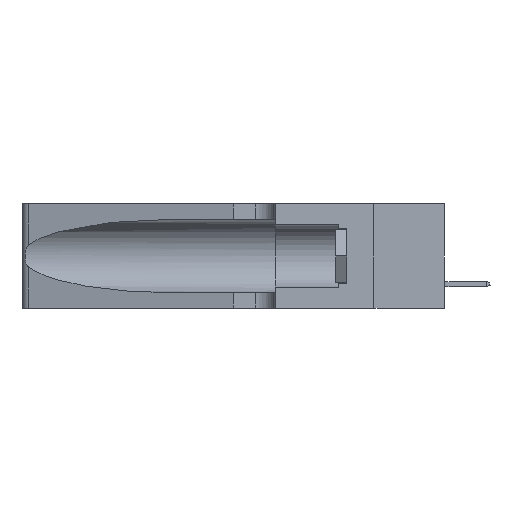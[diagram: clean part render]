
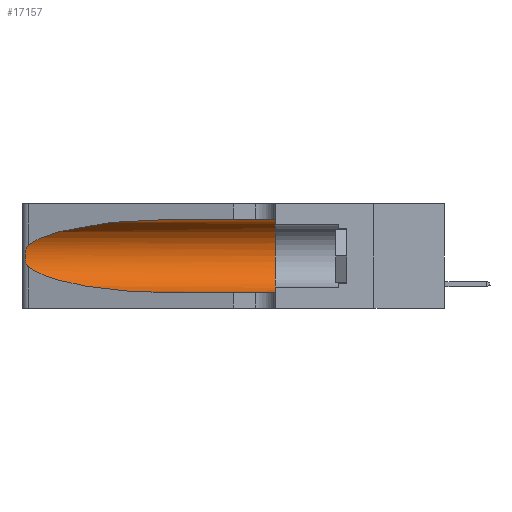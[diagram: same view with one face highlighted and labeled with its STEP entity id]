
A CAD part, left-side view. The second image highlights one B-rep face of the part: STEP entity #17157.
In plain terms, the highlighted cylindrical face has radius 3.308 mm (diameter 6.617 mm), a partial arc.
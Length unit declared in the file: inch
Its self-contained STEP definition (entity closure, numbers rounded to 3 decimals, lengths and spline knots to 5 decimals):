
#274 = EDGE_CURVE ( 'NONE', #12485, #40125, #20227, .T. ) ;
#1479 = EDGE_CURVE ( 'NONE', #34649, #33575, #36860, .T. ) ;
#1816 = DIRECTION ( 'NONE',  ( 0., -1., 0. ) ) ;
#1889 = DIRECTION ( 'NONE',  ( 0., -1., 0. ) ) ;
#3013 = CARTESIAN_POINT ( 'NONE',  ( 0.26017, 1.23833, 0.17102 ) ) ;
#3949 = CARTESIAN_POINT ( 'NONE',  ( 0.25487, 1.22718, 0.14631 ) ) ;
#4555 = CARTESIAN_POINT ( 'NONE',  ( 0.1305, 1.61858, 0.05475 ) ) ;
#5106 = CARTESIAN_POINT ( 'NONE',  ( 0.1305, 0.35, 0.05475 ) ) ;
#5320 = CARTESIAN_POINT ( 'NONE',  ( 0.1305, 1.61858, 0.185 ) ) ;
#5484 = AXIS2_PLACEMENT_3D ( 'NONE', #19870, #16815, #22918 ) ;
#6418 = CARTESIAN_POINT ( 'NONE',  ( 0.25789, 1.23486, 0.15765 ) ) ;
#11421 = CARTESIAN_POINT ( 'NONE',  ( 0.2373, 1.15595, 0.28018 ) ) ;
#11610 = EDGE_CURVE ( 'NONE', #28207, #12485, #38663, .T. ) ;
#12202 = CARTESIAN_POINT ( 'NONE',  ( 0.25787, 1.23484, 0.2124 ) ) ;
#12485 = VERTEX_POINT ( 'NONE', #23934 ) ;
#12583 = CARTESIAN_POINT ( 'NONE',  ( 0.2373, 1.15595, 0.08982 ) ) ;
#13652 = CARTESIAN_POINT ( 'NONE',  ( 0.25555, 1.22994, 0.2215 ) ) ;
#13683 = EDGE_LOOP ( 'NONE', ( #33920, #38998, #14324, #15903, #31220, #14402 ) ) ;
#14324 = ORIENTED_EDGE ( 'NONE', *, *, #1479, .T. ) ;
#14402 = ORIENTED_EDGE ( 'NONE', *, *, #11610, .F. ) ;
#14919 = CARTESIAN_POINT ( 'NONE',  ( 0.25487, 1.22718, 0.14631 ) ) ;
#14974 = CARTESIAN_POINT ( 'NONE',  ( 0.25639, 1.23184, 0.21858 ) ) ;
#14984 =( BOUNDED_CURVE ( )  B_SPLINE_CURVE ( 3, ( #27091, #20641, #11421, #33364 ),
 .UNSPECIFIED., .F., .F. ) 
 B_SPLINE_CURVE_WITH_KNOTS ( ( 4, 4 ),
 ( 1.5708, 2.84003 ),
 .UNSPECIFIED. ) 
 CURVE ( )  GEOMETRIC_REPRESENTATION_ITEM ( )  RATIONAL_B_SPLINE_CURVE ( ( 1., 0.87, 0.87, 1. ) ) 
 REPRESENTATION_ITEM ( '' )  );
#15111 = CARTESIAN_POINT ( 'NONE',  ( 0.25854, 1.2359, 0.20912 ) ) ;
#15767 = CARTESIAN_POINT ( 'NONE',  ( 0.18966, 0.96281, 0.05475 ) ) ;
#15903 = ORIENTED_EDGE ( 'NONE', *, *, #29068, .T. ) ;
#16204 = CYLINDRICAL_SURFACE ( 'NONE', #28271, 0.13025 ) ;
#16815 = DIRECTION ( 'NONE',  ( 0., 1., 0. ) ) ;
#16974 = B_SPLINE_CURVE_WITH_KNOTS ( 'NONE', 3,
 ( #20132, #13652, #14974, #12202, #15111, #31419, #18577, #37722, #3013, #22147, #6418, #31549, #19768, #3949 ),
 .UNSPECIFIED., .F., .F.,
 ( 4, 2, 2, 2, 2, 2, 4 ),
 ( 0., 0.00027, 0.00053, 0.00107, 0.0016, 0.00187, 0.00214 ),
 .UNSPECIFIED. ) ;
#17157 = ADVANCED_FACE ( 'NONE', ( #31435 ), #16204, .F. ) ;
#18577 = CARTESIAN_POINT ( 'NONE',  ( 0.26075, 1.23896, 0.19203 ) ) ;
#19056 = VECTOR ( 'NONE', #1816, 39.37008 ) ;
#19768 = CARTESIAN_POINT ( 'NONE',  ( 0.25555, 1.22993, 0.14849 ) ) ;
#19870 = CARTESIAN_POINT ( 'NONE',  ( 0.1305, 0.35, 0.185 ) ) ;
#20132 = CARTESIAN_POINT ( 'NONE',  ( 0.25487, 1.22718, 0.22369 ) ) ;
#20227 = CIRCLE ( 'NONE', #5484, 0.13025 ) ;
#20641 = CARTESIAN_POINT ( 'NONE',  ( 0.18966, 0.96281, 0.31525 ) ) ;
#20794 = CARTESIAN_POINT ( 'NONE',  ( 0.1305, 1.61858, 0.31525 ) ) ;
#22147 = CARTESIAN_POINT ( 'NONE',  ( 0.25856, 1.23593, 0.16098 ) ) ;
#22849 = VECTOR ( 'NONE', #29687, 39.37008 ) ;
#22918 = DIRECTION ( 'NONE',  ( 0., 0., 1. ) ) ;
#23130 = CARTESIAN_POINT ( 'NONE',  ( 0.25487, 1.22718, 0.14631 ) ) ;
#23930 = DIRECTION ( 'NONE',  ( 0., 0., -1. ) ) ;
#23934 = CARTESIAN_POINT ( 'NONE',  ( 0.1305, 0.35, 0.31525 ) ) ;
#24909 = CARTESIAN_POINT ( 'NONE',  ( 0.1305, 0.72297, 0.05475 ) ) ;
#25099 = EDGE_CURVE ( 'NONE', #25403, #34649, #16974, .T. ) ;
#25403 = VERTEX_POINT ( 'NONE', #30190 ) ;
#27091 = CARTESIAN_POINT ( 'NONE',  ( 0.1305, 0.72297, 0.31525 ) ) ;
#27948 = CARTESIAN_POINT ( 'NONE',  ( 0.1305, 0.72297, 0.31525 ) ) ;
#28207 = VERTEX_POINT ( 'NONE', #27948 ) ;
#28271 = AXIS2_PLACEMENT_3D ( 'NONE', #5320, #1889, #23930 ) ;
#29068 = EDGE_CURVE ( 'NONE', #33575, #40125, #32097, .T. ) ;
#29098 = EDGE_CURVE ( 'NONE', #28207, #25403, #14984, .T. ) ;
#29687 = DIRECTION ( 'NONE',  ( 0., -1., 0. ) ) ;
#30190 = CARTESIAN_POINT ( 'NONE',  ( 0.25487, 1.22718, 0.22369 ) ) ;
#31220 = ORIENTED_EDGE ( 'NONE', *, *, #274, .F. ) ;
#31419 = CARTESIAN_POINT ( 'NONE',  ( 0.26018, 1.23835, 0.19895 ) ) ;
#31435 = FACE_OUTER_BOUND ( 'NONE', #13683, .T. ) ;
#31549 = CARTESIAN_POINT ( 'NONE',  ( 0.25639, 1.23186, 0.15144 ) ) ;
#32097 = LINE ( 'NONE', #4555, #22849 ) ;
#33364 = CARTESIAN_POINT ( 'NONE',  ( 0.25487, 1.22718, 0.22369 ) ) ;
#33575 = VERTEX_POINT ( 'NONE', #33998 ) ;
#33920 = ORIENTED_EDGE ( 'NONE', *, *, #29098, .T. ) ;
#33998 = CARTESIAN_POINT ( 'NONE',  ( 0.1305, 0.72297, 0.05475 ) ) ;
#34649 = VERTEX_POINT ( 'NONE', #14919 ) ;
#36860 =( BOUNDED_CURVE ( )  B_SPLINE_CURVE ( 3, ( #23130, #12583, #15767, #24909 ),
 .UNSPECIFIED., .F., .T. ) 
 B_SPLINE_CURVE_WITH_KNOTS ( ( 4, 4 ),
 ( 3.44316, 4.71239 ),
 .UNSPECIFIED. ) 
 CURVE ( )  GEOMETRIC_REPRESENTATION_ITEM ( )  RATIONAL_B_SPLINE_CURVE ( ( 1., 0.87, 0.87, 1. ) ) 
 REPRESENTATION_ITEM ( '' )  );
#37722 = CARTESIAN_POINT ( 'NONE',  ( 0.26075, 1.23896, 0.178 ) ) ;
#38663 = LINE ( 'NONE', #20794, #19056 ) ;
#38998 = ORIENTED_EDGE ( 'NONE', *, *, #25099, .T. ) ;
#40125 = VERTEX_POINT ( 'NONE', #5106 ) ;
